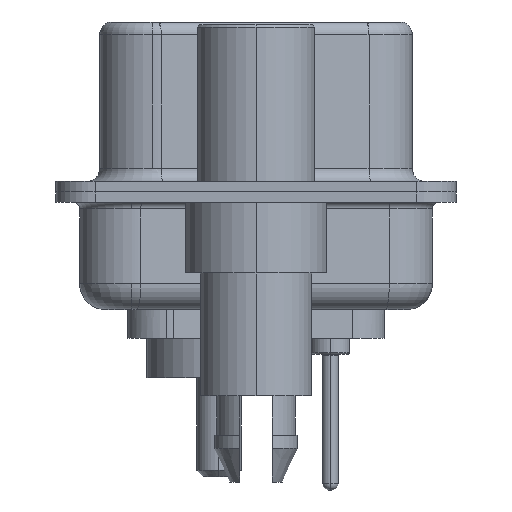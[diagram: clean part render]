
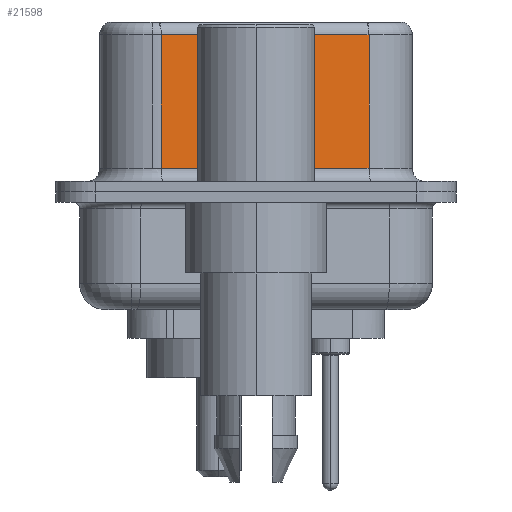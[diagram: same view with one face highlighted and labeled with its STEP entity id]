
A CAD part, left-side view. The second image highlights one B-rep face of the part: STEP entity #21598.
In plain terms, the highlighted planar face has unit normal (-0.985, -0.174, 0).
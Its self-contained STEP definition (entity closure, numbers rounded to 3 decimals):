
#5 = DIRECTION ( 'NONE',  ( -0.174, 0.985, 0. ) ) ;
#64 = ORIENTED_EDGE ( 'NONE', *, *, #13225, .T. ) ;
#1901 = DIRECTION ( 'NONE',  ( 0., 0., -1. ) ) ;
#2772 = ORIENTED_EDGE ( 'NONE', *, *, #23254, .T. ) ;
#3408 = VERTEX_POINT ( 'NONE', #15667 ) ;
#3717 = CARTESIAN_POINT ( 'NONE',  ( 5.132, -4.322, 0.9 ) ) ;
#3881 = VERTEX_POINT ( 'NONE', #3717 ) ;
#4215 = VERTEX_POINT ( 'NONE', #10593 ) ;
#4273 = DIRECTION ( 'NONE',  ( -0.174, 0.985, 0. ) ) ;
#5067 = EDGE_LOOP ( 'NONE', ( #21788, #64, #2772, #20612 ) ) ;
#5631 = CARTESIAN_POINT ( 'NONE',  ( 3.73, 3.628, 6.52 ) ) ;
#5664 = DIRECTION ( 'NONE',  ( 0., 0., -1. ) ) ;
#5681 = DIRECTION ( 'NONE',  ( 0.174, -0.985, 0. ) ) ;
#7797 = VECTOR ( 'NONE', #5681, 1000. ) ;
#8011 = VERTEX_POINT ( 'NONE', #22141 ) ;
#8810 = LINE ( 'NONE', #9574, #18368 ) ;
#9380 = VECTOR ( 'NONE', #5664, 1000. ) ;
#9406 = CARTESIAN_POINT ( 'NONE',  ( 5.132, -4.322, 6.52 ) ) ;
#9574 = CARTESIAN_POINT ( 'NONE',  ( 5.132, -4.322, 6.02 ) ) ;
#10593 = CARTESIAN_POINT ( 'NONE',  ( 3.73, 3.628, 6.02 ) ) ;
#13167 = EDGE_CURVE ( 'NONE', #8011, #3881, #14442, .T. ) ;
#13225 = EDGE_CURVE ( 'NONE', #8011, #4215, #8810, .T. ) ;
#13653 = LINE ( 'NONE', #5631, #18155 ) ;
#14442 = LINE ( 'NONE', #9406, #9380 ) ;
#15667 = CARTESIAN_POINT ( 'NONE',  ( 3.73, 3.628, 0.9 ) ) ;
#15702 = DIRECTION ( 'NONE',  ( 0.985, 0.174, 0. ) ) ;
#16935 = CARTESIAN_POINT ( 'NONE',  ( 5.132, -4.322, 6.52 ) ) ;
#17097 = CARTESIAN_POINT ( 'NONE',  ( 5.132, -4.322, 0.9 ) ) ;
#18155 = VECTOR ( 'NONE', #1901, 1000. ) ;
#18368 = VECTOR ( 'NONE', #5, 1000. ) ;
#18984 = PLANE ( 'NONE',  #23097 ) ;
#19609 = EDGE_CURVE ( 'NONE', #3408, #3881, #23675, .T. ) ;
#20587 = FACE_OUTER_BOUND ( 'NONE', #5067, .T. ) ;
#20612 = ORIENTED_EDGE ( 'NONE', *, *, #19609, .T. ) ;
#21598 = ADVANCED_FACE ( 'NONE', ( #20587 ), #18984, .F. ) ;
#21788 = ORIENTED_EDGE ( 'NONE', *, *, #13167, .F. ) ;
#22141 = CARTESIAN_POINT ( 'NONE',  ( 5.132, -4.322, 6.02 ) ) ;
#23097 = AXIS2_PLACEMENT_3D ( 'NONE', #16935, #15702, #4273 ) ;
#23254 = EDGE_CURVE ( 'NONE', #4215, #3408, #13653, .T. ) ;
#23675 = LINE ( 'NONE', #17097, #7797 ) ;
